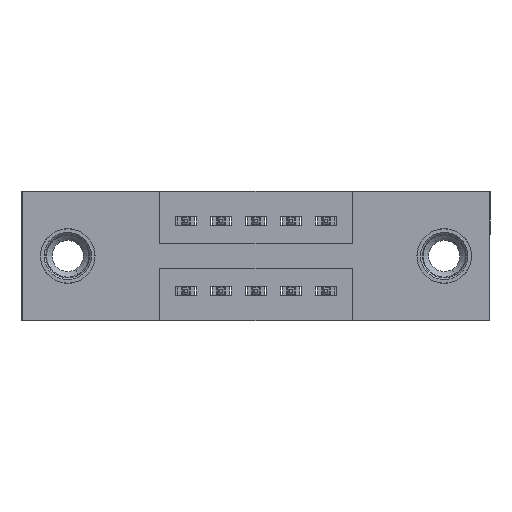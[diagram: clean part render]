
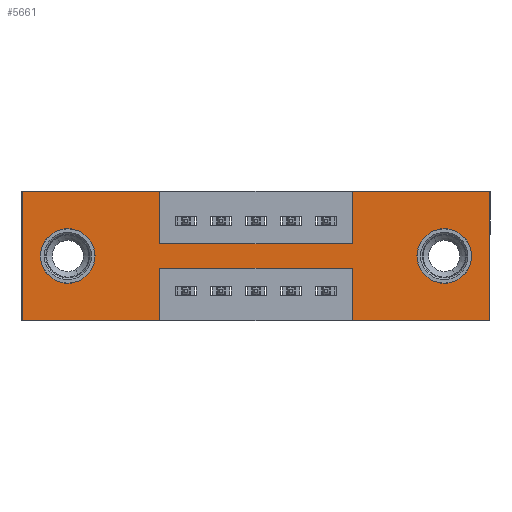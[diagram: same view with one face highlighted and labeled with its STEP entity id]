
A CAD part, front view. The second image highlights one B-rep face of the part: STEP entity #5661.
In plain terms, the highlighted planar face has unit normal (0, -1, 0).
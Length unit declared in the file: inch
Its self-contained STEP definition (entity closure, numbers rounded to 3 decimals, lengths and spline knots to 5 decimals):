
#139 = FACE_OUTER_BOUND ( 'NONE', #3695, .T. ) ;
#194 = ORIENTED_EDGE ( 'NONE', *, *, #1987, .F. ) ;
#240 = ORIENTED_EDGE ( 'NONE', *, *, #1378, .F. ) ;
#276 = VECTOR ( 'NONE', #6752, 39.37008 ) ;
#388 = ORIENTED_EDGE ( 'NONE', *, *, #7690, .T. ) ;
#469 = CARTESIAN_POINT ( 'NONE',  ( 0.3925, 0., -0.15 ) ) ;
#561 = DIRECTION ( 'NONE',  ( 0., 0., -1. ) ) ;
#565 = LINE ( 'NONE', #10463, #7538 ) ;
#612 = DIRECTION ( 'NONE',  ( -1., 0., 0. ) ) ;
#630 = DIRECTION ( 'NONE',  ( 0., 0., -1. ) ) ;
#641 = CARTESIAN_POINT ( 'NONE',  ( 1.335, 0., 0. ) ) ;
#719 = LINE ( 'NONE', #641, #5152 ) ;
#966 = EDGE_CURVE ( 'NONE', #8656, #2808, #6122, .T. ) ;
#1032 = LINE ( 'NONE', #4237, #9876 ) ;
#1128 = DIRECTION ( 'NONE',  ( 0., 0., 1. ) ) ;
#1293 = CARTESIAN_POINT ( 'NONE',  ( 0., 0., 0. ) ) ;
#1373 = VERTEX_POINT ( 'NONE', #8038 ) ;
#1378 = EDGE_CURVE ( 'NONE', #1968, #1457, #2303, .T. ) ;
#1406 = VERTEX_POINT ( 'NONE', #3809 ) ;
#1417 = ORIENTED_EDGE ( 'NONE', *, *, #3323, .T. ) ;
#1439 = VECTOR ( 'NONE', #3181, 39.37008 ) ;
#1457 = VERTEX_POINT ( 'NONE', #3178 ) ;
#1542 = VERTEX_POINT ( 'NONE', #5950 ) ;
#1563 = LINE ( 'NONE', #7425, #5916 ) ;
#1612 = DIRECTION ( 'NONE',  ( -1., 0., 0. ) ) ;
#1614 = PLANE ( 'NONE',  #8443 ) ;
#1791 = VERTEX_POINT ( 'NONE', #10920 ) ;
#1968 = VERTEX_POINT ( 'NONE', #7700 ) ;
#1987 = EDGE_CURVE ( 'NONE', #2761, #5655, #565, .T. ) ;
#2223 = EDGE_CURVE ( 'NONE', #1406, #1373, #719, .T. ) ;
#2303 = LINE ( 'NONE', #10767, #8844 ) ;
#2310 = ORIENTED_EDGE ( 'NONE', *, *, #3617, .F. ) ;
#2430 = LINE ( 'NONE', #5038, #276 ) ;
#2463 = AXIS2_PLACEMENT_3D ( 'NONE', #2894, #9793, #7814 ) ;
#2672 = DIRECTION ( 'NONE',  ( 0., 1., 0. ) ) ;
#2761 = VERTEX_POINT ( 'NONE', #5341 ) ;
#2808 = VERTEX_POINT ( 'NONE', #8288 ) ;
#2894 = CARTESIAN_POINT ( 'NONE',  ( 0.13, 0., -0.185 ) ) ;
#3013 = VERTEX_POINT ( 'NONE', #5217 ) ;
#3178 = CARTESIAN_POINT ( 'NONE',  ( 0.9425, 0., 0. ) ) ;
#3181 = DIRECTION ( 'NONE',  ( 1., 0., 0. ) ) ;
#3323 = EDGE_CURVE ( 'NONE', #8415, #1542, #9072, .T. ) ;
#3358 = ORIENTED_EDGE ( 'NONE', *, *, #9528, .F. ) ;
#3363 = CARTESIAN_POINT ( 'NONE',  ( 0.3925, 0., -0.37 ) ) ;
#3401 = DIRECTION ( 'NONE',  ( 0., -1., 0. ) ) ;
#3617 = EDGE_CURVE ( 'NONE', #5655, #1791, #1563, .T. ) ;
#3621 = ORIENTED_EDGE ( 'NONE', *, *, #9388, .F. ) ;
#3695 = EDGE_LOOP ( 'NONE', ( #3621, #3358, #5371, #7519, #7521, #10912, #240, #6107, #8362, #2310, #194, #9932 ) ) ;
#3809 = CARTESIAN_POINT ( 'NONE',  ( 1.335, 0., 0. ) ) ;
#4046 = VECTOR ( 'NONE', #4818, 39.37008 ) ;
#4237 = CARTESIAN_POINT ( 'NONE',  ( 0., 0., -0.37 ) ) ;
#4263 = DIRECTION ( 'NONE',  ( 0., 0., -1. ) ) ;
#4306 = DIRECTION ( 'NONE',  ( 0., 1., 0. ) ) ;
#4393 = CARTESIAN_POINT ( 'NONE',  ( 1.205, 0., -0.185 ) ) ;
#4533 = VERTEX_POINT ( 'NONE', #8532 ) ;
#4818 = DIRECTION ( 'NONE',  ( 1., 0., 0. ) ) ;
#4831 = CARTESIAN_POINT ( 'NONE',  ( 0.3925, 0., -0.37 ) ) ;
#4864 = DIRECTION ( 'NONE',  ( -1., 0., 0. ) ) ;
#4939 = EDGE_LOOP ( 'NONE', ( #1417, #388 ) ) ;
#4969 = VECTOR ( 'NONE', #612, 39.37008 ) ;
#5038 = CARTESIAN_POINT ( 'NONE',  ( 0.3925, 0., 0. ) ) ;
#5152 = VECTOR ( 'NONE', #561, 39.37008 ) ;
#5162 = CARTESIAN_POINT ( 'NONE',  ( 1.205, 0., -0.107 ) ) ;
#5217 = CARTESIAN_POINT ( 'NONE',  ( 0.3925, 0., -0.15 ) ) ;
#5258 = LINE ( 'NONE', #8213, #9447 ) ;
#5341 = CARTESIAN_POINT ( 'NONE',  ( 0., 0., -0.37 ) ) ;
#5371 = ORIENTED_EDGE ( 'NONE', *, *, #5535, .F. ) ;
#5535 = EDGE_CURVE ( 'NONE', #10030, #10076, #8475, .T. ) ;
#5655 = VERTEX_POINT ( 'NONE', #7601 ) ;
#5661 = ADVANCED_FACE ( 'NONE', ( #9119, #9376, #139 ), #1614, .T. ) ;
#5915 = DIRECTION ( 'NONE',  ( 0., 1., 0. ) ) ;
#5916 = VECTOR ( 'NONE', #10713, 39.37008 ) ;
#5950 = CARTESIAN_POINT ( 'NONE',  ( 1.205, 0., -0.263 ) ) ;
#5982 = VECTOR ( 'NONE', #9166, 39.37008 ) ;
#6083 = CIRCLE ( 'NONE', #10122, 0.078 ) ;
#6107 = ORIENTED_EDGE ( 'NONE', *, *, #10096, .F. ) ;
#6122 = CIRCLE ( 'NONE', #2463, 0.078 ) ;
#6287 = EDGE_CURVE ( 'NONE', #1791, #3013, #2430, .T. ) ;
#6293 = ORIENTED_EDGE ( 'NONE', *, *, #966, .T. ) ;
#6428 = EDGE_CURVE ( 'NONE', #1373, #10030, #1032, .T. ) ;
#6577 = LINE ( 'NONE', #4831, #10987 ) ;
#6752 = DIRECTION ( 'NONE',  ( 0., 0., -1. ) ) ;
#7217 = LINE ( 'NONE', #10059, #4969 ) ;
#7425 = CARTESIAN_POINT ( 'NONE',  ( 0., 0., 0. ) ) ;
#7459 = ORIENTED_EDGE ( 'NONE', *, *, #10318, .T. ) ;
#7519 = ORIENTED_EDGE ( 'NONE', *, *, #6428, .F. ) ;
#7521 = ORIENTED_EDGE ( 'NONE', *, *, #2223, .F. ) ;
#7538 = VECTOR ( 'NONE', #1128, 39.37008 ) ;
#7601 = CARTESIAN_POINT ( 'NONE',  ( 0., 0., 0. ) ) ;
#7690 = EDGE_CURVE ( 'NONE', #1542, #8415, #10494, .T. ) ;
#7700 = CARTESIAN_POINT ( 'NONE',  ( 0.9425, 0., -0.15 ) ) ;
#7717 = VERTEX_POINT ( 'NONE', #3363 ) ;
#7801 = CARTESIAN_POINT ( 'NONE',  ( 0.13, 0., -0.185 ) ) ;
#7814 = DIRECTION ( 'NONE',  ( 0., 0., 1. ) ) ;
#8038 = CARTESIAN_POINT ( 'NONE',  ( 1.335, 0., -0.37 ) ) ;
#8213 = CARTESIAN_POINT ( 'NONE',  ( 0., 0., -0.37 ) ) ;
#8288 = CARTESIAN_POINT ( 'NONE',  ( 0.13, 0., -0.263 ) ) ;
#8341 = CARTESIAN_POINT ( 'NONE',  ( 0.9425, 0., -0.37 ) ) ;
#8362 = ORIENTED_EDGE ( 'NONE', *, *, #6287, .F. ) ;
#8415 = VERTEX_POINT ( 'NONE', #5162 ) ;
#8443 = AXIS2_PLACEMENT_3D ( 'NONE', #8479, #3401, #9307 ) ;
#8475 = LINE ( 'NONE', #8341, #5982 ) ;
#8479 = CARTESIAN_POINT ( 'NONE',  ( 0., 0., -0.37 ) ) ;
#8532 = CARTESIAN_POINT ( 'NONE',  ( 0.3925, 0., -0.22 ) ) ;
#8558 = LINE ( 'NONE', #469, #1439 ) ;
#8637 = DIRECTION ( 'NONE',  ( 0., 0., 1. ) ) ;
#8656 = VERTEX_POINT ( 'NONE', #9010 ) ;
#8681 = EDGE_CURVE ( 'NONE', #7717, #2761, #5258, .T. ) ;
#8844 = VECTOR ( 'NONE', #11047, 39.37008 ) ;
#8982 = AXIS2_PLACEMENT_3D ( 'NONE', #4393, #4306, #4263 ) ;
#9010 = CARTESIAN_POINT ( 'NONE',  ( 0.13, 0., -0.107 ) ) ;
#9072 = CIRCLE ( 'NONE', #8982, 0.078 ) ;
#9119 = FACE_BOUND ( 'NONE', #4939, .T. ) ;
#9166 = DIRECTION ( 'NONE',  ( 0., 0., 1. ) ) ;
#9307 = DIRECTION ( 'NONE',  ( 0., 0., -1. ) ) ;
#9376 = FACE_BOUND ( 'NONE', #9766, .T. ) ;
#9388 = EDGE_CURVE ( 'NONE', #4533, #7717, #6577, .T. ) ;
#9447 = VECTOR ( 'NONE', #4864, 39.37008 ) ;
#9528 = EDGE_CURVE ( 'NONE', #10076, #4533, #7217, .T. ) ;
#9766 = EDGE_LOOP ( 'NONE', ( #6293, #7459 ) ) ;
#9793 = DIRECTION ( 'NONE',  ( 0., 1., 0. ) ) ;
#9838 = CARTESIAN_POINT ( 'NONE',  ( 0.9425, 0., -0.37 ) ) ;
#9876 = VECTOR ( 'NONE', #1612, 39.37008 ) ;
#9932 = ORIENTED_EDGE ( 'NONE', *, *, #8681, .F. ) ;
#10006 = EDGE_CURVE ( 'NONE', #1457, #1406, #10736, .T. ) ;
#10030 = VERTEX_POINT ( 'NONE', #9838 ) ;
#10059 = CARTESIAN_POINT ( 'NONE',  ( 0.3925, 0., -0.22 ) ) ;
#10076 = VERTEX_POINT ( 'NONE', #10737 ) ;
#10096 = EDGE_CURVE ( 'NONE', #3013, #1968, #8558, .T. ) ;
#10122 = AXIS2_PLACEMENT_3D ( 'NONE', #7801, #2672, #8637 ) ;
#10318 = EDGE_CURVE ( 'NONE', #2808, #8656, #6083, .T. ) ;
#10463 = CARTESIAN_POINT ( 'NONE',  ( 0., 0., 0. ) ) ;
#10494 = CIRCLE ( 'NONE', #11079, 0.078 ) ;
#10673 = DIRECTION ( 'NONE',  ( 0., 0., -1. ) ) ;
#10713 = DIRECTION ( 'NONE',  ( 1., 0., 0. ) ) ;
#10736 = LINE ( 'NONE', #1293, #4046 ) ;
#10737 = CARTESIAN_POINT ( 'NONE',  ( 0.9425, 0., -0.22 ) ) ;
#10767 = CARTESIAN_POINT ( 'NONE',  ( 0.9425, 0., 0. ) ) ;
#10899 = CARTESIAN_POINT ( 'NONE',  ( 1.205, 0., -0.185 ) ) ;
#10912 = ORIENTED_EDGE ( 'NONE', *, *, #10006, .F. ) ;
#10920 = CARTESIAN_POINT ( 'NONE',  ( 0.3925, 0., 0. ) ) ;
#10987 = VECTOR ( 'NONE', #10673, 39.37008 ) ;
#11047 = DIRECTION ( 'NONE',  ( 0., 0., 1. ) ) ;
#11079 = AXIS2_PLACEMENT_3D ( 'NONE', #10899, #5915, #630 ) ;
